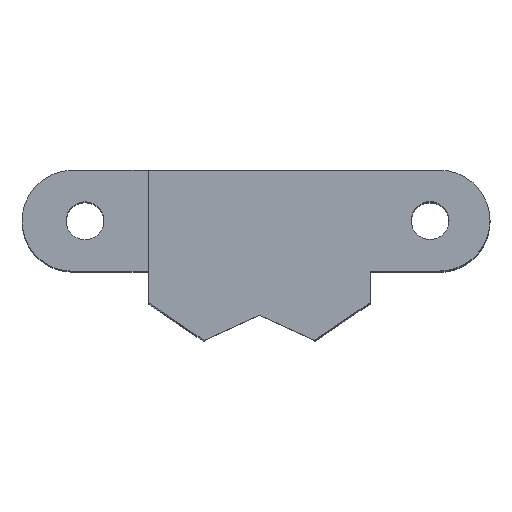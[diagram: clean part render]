
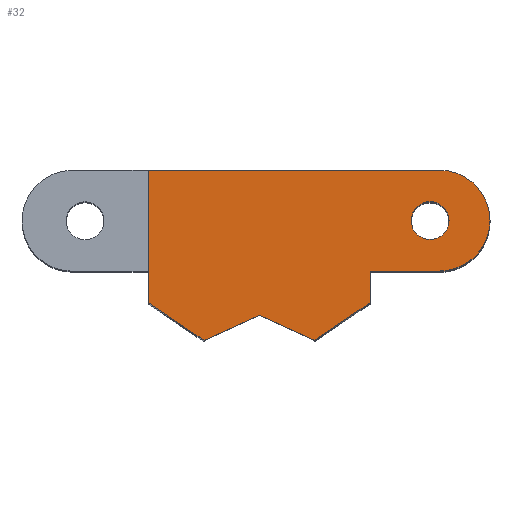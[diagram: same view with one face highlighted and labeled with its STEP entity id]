
A CAD part, top view. The second image highlights one B-rep face of the part: STEP entity #32.
In plain terms, the highlighted planar face has unit normal (0, 0, 1).
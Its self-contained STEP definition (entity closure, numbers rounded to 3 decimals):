
#32 = ADVANCED_FACE ( 'NONE', ( #802, #1496 ), #1481, .T. ) ;
#127 = VERTEX_POINT ( 'NONE', #712 ) ;
#163 = VERTEX_POINT ( 'NONE', #1874 ) ;
#173 = VERTEX_POINT ( 'NONE', #1739 ) ;
#226 = EDGE_LOOP ( 'NONE', ( #1129, #2036, #2160, #1793, #406, #1091, #412, #1648, #558, #872 ) ) ;
#228 = CIRCLE ( 'NONE', #1709, 4. ) ;
#278 = VERTEX_POINT ( 'NONE', #2090 ) ;
#317 = CARTESIAN_POINT ( 'NONE',  ( -8.8, 11.5, 33. ) ) ;
#352 = CARTESIAN_POINT ( 'NONE',  ( 15.05, 7.5, 33. ) ) ;
#360 = AXIS2_PLACEMENT_3D ( 'NONE', #2191, #648, #1854 ) ;
#370 = AXIS2_PLACEMENT_3D ( 'NONE', #1844, #1472, #1509 ) ;
#406 = ORIENTED_EDGE ( 'NONE', *, *, #617, .T. ) ;
#412 = ORIENTED_EDGE ( 'NONE', *, *, #621, .T. ) ;
#467 = DIRECTION ( 'NONE',  ( 1., 0., 0. ) ) ;
#484 = VECTOR ( 'NONE', #1740, 1000. ) ;
#489 = EDGE_CURVE ( 'NONE', #127, #1242, #830, .T. ) ;
#521 = DIRECTION ( 'NONE',  ( 1., 0., 0. ) ) ;
#532 = VERTEX_POINT ( 'NONE', #1347 ) ;
#548 = EDGE_CURVE ( 'NONE', #173, #1165, #1999, .T. ) ;
#558 = ORIENTED_EDGE ( 'NONE', *, *, #624, .T. ) ;
#569 = ORIENTED_EDGE ( 'NONE', *, *, #910, .F. ) ;
#580 = DIRECTION ( 'NONE',  ( 0.909, 0.417, 0. ) ) ;
#604 = CARTESIAN_POINT ( 'NONE',  ( 4.363, -2., 33. ) ) ;
#611 = CARTESIAN_POINT ( 'NONE',  ( -8.8, 1., 33. ) ) ;
#617 = EDGE_CURVE ( 'NONE', #1407, #173, #813, .T. ) ;
#621 = EDGE_CURVE ( 'NONE', #1165, #278, #1998, .T. ) ;
#624 = EDGE_CURVE ( 'NONE', #1798, #532, #967, .T. ) ;
#629 = DIRECTION ( 'NONE',  ( 1., 0., 0. ) ) ;
#647 = CARTESIAN_POINT ( 'NONE',  ( -4.363, -2., 33. ) ) ;
#648 = DIRECTION ( 'NONE',  ( 0., 0., 1. ) ) ;
#675 = VECTOR ( 'NONE', #1315, 1000. ) ;
#712 = CARTESIAN_POINT ( 'NONE',  ( 8.8, 3.5, 33. ) ) ;
#725 = AXIS2_PLACEMENT_3D ( 'NONE', #868, #1202, #521 ) ;
#741 = LINE ( 'NONE', #1424, #484 ) ;
#783 = VECTOR ( 'NONE', #580, 1000. ) ;
#802 = FACE_OUTER_BOUND ( 'NONE', #226, .T. ) ;
#813 = LINE ( 'NONE', #611, #2131 ) ;
#830 = LINE ( 'NONE', #1532, #675 ) ;
#846 = DIRECTION ( 'NONE',  ( 0.828, -0.56, 0. ) ) ;
#868 = CARTESIAN_POINT ( 'NONE',  ( 14.3, 7.5, 33. ) ) ;
#872 = ORIENTED_EDGE ( 'NONE', *, *, #1085, .T. ) ;
#910 = EDGE_CURVE ( 'NONE', #163, #1573, #1338, .T. ) ;
#924 = VECTOR ( 'NONE', #846, 1000. ) ;
#926 = EDGE_CURVE ( 'NONE', #1242, #1393, #1623, .T. ) ;
#961 = VERTEX_POINT ( 'NONE', #1917 ) ;
#967 = LINE ( 'NONE', #1973, #2034 ) ;
#989 = CARTESIAN_POINT ( 'NONE',  ( -4.363, -2., 33. ) ) ;
#994 = AXIS2_PLACEMENT_3D ( 'NONE', #2162, #1139, #629 ) ;
#995 = DIRECTION ( 'NONE',  ( -1., 0., 0. ) ) ;
#1085 = EDGE_CURVE ( 'NONE', #532, #127, #741, .T. ) ;
#1091 = ORIENTED_EDGE ( 'NONE', *, *, #548, .T. ) ;
#1119 = CARTESIAN_POINT ( 'NONE',  ( -8.8, 11.5, 33. ) ) ;
#1129 = ORIENTED_EDGE ( 'NONE', *, *, #489, .T. ) ;
#1139 = DIRECTION ( 'NONE',  ( 0., 0., 1. ) ) ;
#1153 = CARTESIAN_POINT ( 'NONE',  ( 18.3, 7.5, 33. ) ) ;
#1165 = VERTEX_POINT ( 'NONE', #647 ) ;
#1189 = EDGE_CURVE ( 'NONE', #961, #1407, #1659, .T. ) ;
#1202 = DIRECTION ( 'NONE',  ( 0., 0., 1. ) ) ;
#1228 = ORIENTED_EDGE ( 'NONE', *, *, #1420, .F. ) ;
#1242 = VERTEX_POINT ( 'NONE', #1324 ) ;
#1248 = EDGE_CURVE ( 'NONE', #1393, #961, #228, .T. ) ;
#1249 = DIRECTION ( 'NONE',  ( 0.909, -0.417, 0. ) ) ;
#1314 = DIRECTION ( 'NONE',  ( 0., -1., 0. ) ) ;
#1315 = DIRECTION ( 'NONE',  ( 1., 0., 0. ) ) ;
#1324 = CARTESIAN_POINT ( 'NONE',  ( 14.3, 3.5, 33. ) ) ;
#1333 = EDGE_LOOP ( 'NONE', ( #1228, #569 ) ) ;
#1338 = CIRCLE ( 'NONE', #360, 1.5 ) ;
#1343 = CARTESIAN_POINT ( 'NONE',  ( 14.3, 7.5, 33. ) ) ;
#1347 = CARTESIAN_POINT ( 'NONE',  ( 8.8, 1., 33. ) ) ;
#1393 = VERTEX_POINT ( 'NONE', #1153 ) ;
#1407 = VERTEX_POINT ( 'NONE', #1119 ) ;
#1420 = EDGE_CURVE ( 'NONE', #1573, #163, #1561, .T. ) ;
#1424 = CARTESIAN_POINT ( 'NONE',  ( 8.8, 1., 33. ) ) ;
#1472 = DIRECTION ( 'NONE',  ( 0., 0., 1. ) ) ;
#1481 = PLANE ( 'NONE',  #994 ) ;
#1484 = VECTOR ( 'NONE', #1249, 1000. ) ;
#1493 = CARTESIAN_POINT ( 'NONE',  ( -4.363, -2., 33. ) ) ;
#1496 = FACE_BOUND ( 'NONE', #1333, .T. ) ;
#1509 = DIRECTION ( 'NONE',  ( 1., 0., 0. ) ) ;
#1532 = CARTESIAN_POINT ( 'NONE',  ( 8.8, 3.5, 33. ) ) ;
#1561 = CIRCLE ( 'NONE', #370, 1.5 ) ;
#1573 = VERTEX_POINT ( 'NONE', #352 ) ;
#1578 = CARTESIAN_POINT ( 'NONE',  ( 0., 0., 33. ) ) ;
#1623 = CIRCLE ( 'NONE', #725, 4. ) ;
#1648 = ORIENTED_EDGE ( 'NONE', *, *, #2141, .T. ) ;
#1659 = LINE ( 'NONE', #317, #2031 ) ;
#1709 = AXIS2_PLACEMENT_3D ( 'NONE', #1343, #2007, #467 ) ;
#1739 = CARTESIAN_POINT ( 'NONE',  ( -8.8, 1., 33. ) ) ;
#1740 = DIRECTION ( 'NONE',  ( 0., 1., 0. ) ) ;
#1793 = ORIENTED_EDGE ( 'NONE', *, *, #1189, .T. ) ;
#1798 = VERTEX_POINT ( 'NONE', #604 ) ;
#1844 = CARTESIAN_POINT ( 'NONE',  ( 13.55, 7.5, 33. ) ) ;
#1854 = DIRECTION ( 'NONE',  ( 1., 0., 0. ) ) ;
#1874 = CARTESIAN_POINT ( 'NONE',  ( 12.05, 7.5, 33. ) ) ;
#1901 = LINE ( 'NONE', #1578, #1484 ) ;
#1917 = CARTESIAN_POINT ( 'NONE',  ( 14.3, 11.5, 33. ) ) ;
#1973 = CARTESIAN_POINT ( 'NONE',  ( 4.363, -2., 33. ) ) ;
#1998 = LINE ( 'NONE', #1493, #783 ) ;
#1999 = LINE ( 'NONE', #989, #924 ) ;
#2007 = DIRECTION ( 'NONE',  ( 0., 0., 1. ) ) ;
#2031 = VECTOR ( 'NONE', #995, 1000. ) ;
#2034 = VECTOR ( 'NONE', #2122, 1000. ) ;
#2036 = ORIENTED_EDGE ( 'NONE', *, *, #926, .T. ) ;
#2090 = CARTESIAN_POINT ( 'NONE',  ( 0., 0., 33. ) ) ;
#2122 = DIRECTION ( 'NONE',  ( 0.828, 0.56, 0. ) ) ;
#2131 = VECTOR ( 'NONE', #1314, 1000. ) ;
#2141 = EDGE_CURVE ( 'NONE', #278, #1798, #1901, .T. ) ;
#2160 = ORIENTED_EDGE ( 'NONE', *, *, #1248, .T. ) ;
#2162 = CARTESIAN_POINT ( 'NONE',  ( 0., 0., 33. ) ) ;
#2191 = CARTESIAN_POINT ( 'NONE',  ( 13.55, 7.5, 33. ) ) ;
